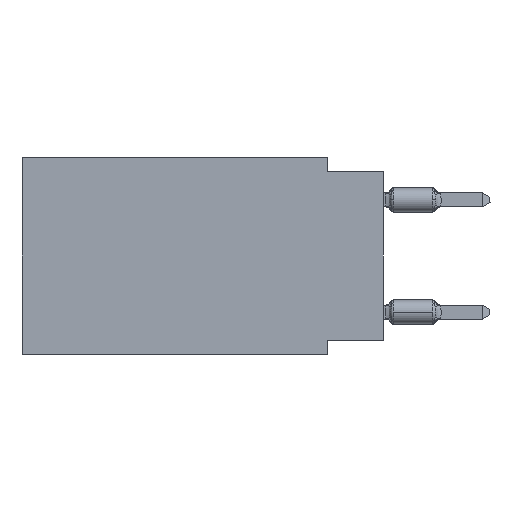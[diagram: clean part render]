
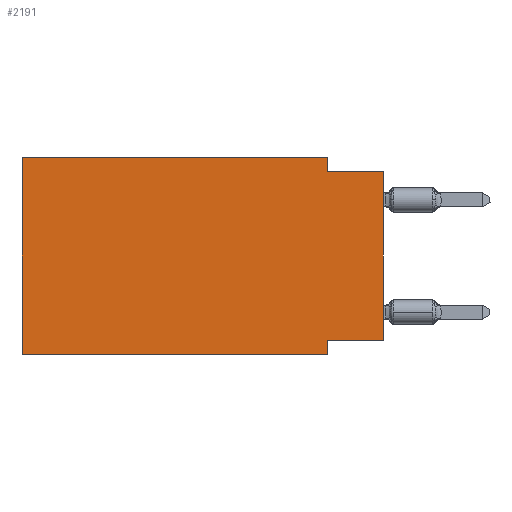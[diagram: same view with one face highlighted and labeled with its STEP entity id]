
A CAD part, left-side view. The second image highlights one B-rep face of the part: STEP entity #2191.
In plain terms, the highlighted planar face has unit normal (-1, 0, 0).
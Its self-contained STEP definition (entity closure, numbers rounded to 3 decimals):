
#37 = DIRECTION ( 'NONE',  ( 0., 0., -1. ) ) ;
#945 = CARTESIAN_POINT ( 'NONE',  ( 0., 2.54, 0. ) ) ;
#1116 = VERTEX_POINT ( 'NONE', #18599 ) ;
#1142 = EDGE_CURVE ( 'NONE', #10525, #7036, #21269, .T. ) ;
#1355 = VERTEX_POINT ( 'NONE', #27703 ) ;
#1394 = LINE ( 'NONE', #26755, #2521 ) ;
#1928 = ORIENTED_EDGE ( 'NONE', *, *, #18994, .T. ) ;
#2086 = EDGE_CURVE ( 'NONE', #14915, #1355, #11244, .T. ) ;
#2191 = ADVANCED_FACE ( 'NONE', ( #23038 ), #22759, .F. ) ;
#2252 = DIRECTION ( 'NONE',  ( 0., 1., 0. ) ) ;
#2294 = VECTOR ( 'NONE', #22584, 1000. ) ;
#2444 = CARTESIAN_POINT ( 'NONE',  ( 0., 2.54, -8.89 ) ) ;
#2521 = VECTOR ( 'NONE', #9983, 1000. ) ;
#2731 = ORIENTED_EDGE ( 'NONE', *, *, #15673, .F. ) ;
#2929 = VECTOR ( 'NONE', #16871, 1000. ) ;
#3281 = CARTESIAN_POINT ( 'NONE',  ( 0., 2.54, -8.255 ) ) ;
#3546 = VECTOR ( 'NONE', #15624, 1000. ) ;
#5014 = CARTESIAN_POINT ( 'NONE',  ( 0., 16.383, 0. ) ) ;
#5534 = CARTESIAN_POINT ( 'NONE',  ( 0., 2.54, -8.89 ) ) ;
#5833 = VERTEX_POINT ( 'NONE', #5534 ) ;
#7036 = VERTEX_POINT ( 'NONE', #3281 ) ;
#8111 = DIRECTION ( 'NONE',  ( 1., 0., 0. ) ) ;
#9082 = DIRECTION ( 'NONE',  ( 0., -1., 0. ) ) ;
#9983 = DIRECTION ( 'NONE',  ( 0., 0., 1. ) ) ;
#10368 = ORIENTED_EDGE ( 'NONE', *, *, #19433, .F. ) ;
#10525 = VERTEX_POINT ( 'NONE', #27733 ) ;
#10607 = VECTOR ( 'NONE', #9082, 1000. ) ;
#11244 = LINE ( 'NONE', #945, #3546 ) ;
#11899 = VERTEX_POINT ( 'NONE', #27560 ) ;
#12066 = ORIENTED_EDGE ( 'NONE', *, *, #21142, .F. ) ;
#12097 = CARTESIAN_POINT ( 'NONE',  ( 0., 16.383, 0. ) ) ;
#12528 = VECTOR ( 'NONE', #2252, 1000. ) ;
#12546 = CARTESIAN_POINT ( 'NONE',  ( 0., 0., -8.255 ) ) ;
#12928 = CARTESIAN_POINT ( 'NONE',  ( 0., 16.383, 0. ) ) ;
#13043 = VERTEX_POINT ( 'NONE', #12097 ) ;
#13062 = EDGE_LOOP ( 'NONE', ( #25053, #12066, #21576, #10368, #13826, #1928, #2731, #17464 ) ) ;
#13826 = ORIENTED_EDGE ( 'NONE', *, *, #14206, .F. ) ;
#14010 = LINE ( 'NONE', #5014, #2294 ) ;
#14206 = EDGE_CURVE ( 'NONE', #11899, #13043, #14010, .T. ) ;
#14504 = VECTOR ( 'NONE', #37, 1000. ) ;
#14915 = VERTEX_POINT ( 'NONE', #15368 ) ;
#15368 = CARTESIAN_POINT ( 'NONE',  ( 0., 2.54, 0. ) ) ;
#15624 = DIRECTION ( 'NONE',  ( 0., 0., -1. ) ) ;
#15673 = EDGE_CURVE ( 'NONE', #7036, #5833, #25963, .T. ) ;
#16708 = CARTESIAN_POINT ( 'NONE',  ( 0., 16.383, 0. ) ) ;
#16825 = VECTOR ( 'NONE', #26906, 1000. ) ;
#16871 = DIRECTION ( 'NONE',  ( 0., -1., 0. ) ) ;
#17464 = ORIENTED_EDGE ( 'NONE', *, *, #1142, .F. ) ;
#18590 = LINE ( 'NONE', #20704, #16825 ) ;
#18599 = CARTESIAN_POINT ( 'NONE',  ( 0., 0., -0.635 ) ) ;
#18994 = EDGE_CURVE ( 'NONE', #11899, #5833, #18590, .T. ) ;
#19433 = EDGE_CURVE ( 'NONE', #13043, #14915, #23468, .T. ) ;
#19782 = LINE ( 'NONE', #24416, #10607 ) ;
#20704 = CARTESIAN_POINT ( 'NONE',  ( 0., 16.383, -8.89 ) ) ;
#21068 = DIRECTION ( 'NONE',  ( 0., 0., -1. ) ) ;
#21142 = EDGE_CURVE ( 'NONE', #1355, #1116, #19782, .T. ) ;
#21269 = LINE ( 'NONE', #12546, #12528 ) ;
#21454 = EDGE_CURVE ( 'NONE', #10525, #1116, #1394, .T. ) ;
#21576 = ORIENTED_EDGE ( 'NONE', *, *, #2086, .F. ) ;
#22584 = DIRECTION ( 'NONE',  ( 0., 0., 1. ) ) ;
#22759 = PLANE ( 'NONE',  #27410 ) ;
#23038 = FACE_OUTER_BOUND ( 'NONE', #13062, .T. ) ;
#23468 = LINE ( 'NONE', #12928, #2929 ) ;
#24416 = CARTESIAN_POINT ( 'NONE',  ( 0., 0., -0.635 ) ) ;
#25053 = ORIENTED_EDGE ( 'NONE', *, *, #21454, .T. ) ;
#25963 = LINE ( 'NONE', #2444, #14504 ) ;
#26755 = CARTESIAN_POINT ( 'NONE',  ( 0., 0., 0. ) ) ;
#26906 = DIRECTION ( 'NONE',  ( 0., -1., 0. ) ) ;
#27410 = AXIS2_PLACEMENT_3D ( 'NONE', #16708, #8111, #21068 ) ;
#27560 = CARTESIAN_POINT ( 'NONE',  ( 0., 16.383, -8.89 ) ) ;
#27703 = CARTESIAN_POINT ( 'NONE',  ( 0., 2.54, -0.635 ) ) ;
#27733 = CARTESIAN_POINT ( 'NONE',  ( 0., 0., -8.255 ) ) ;
